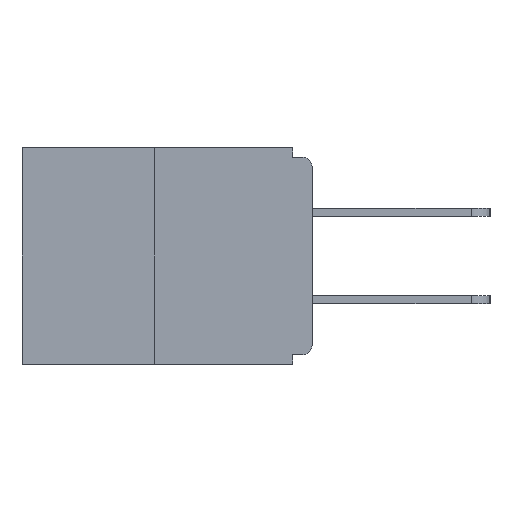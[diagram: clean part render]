
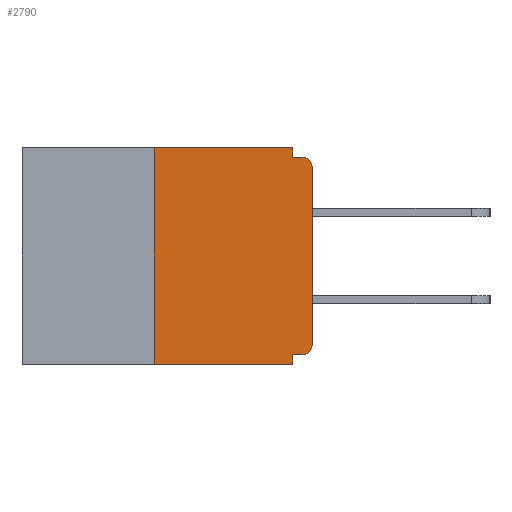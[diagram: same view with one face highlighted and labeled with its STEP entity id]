
A CAD part, left-side view. The second image highlights one B-rep face of the part: STEP entity #2790.
In plain terms, the highlighted planar face has unit normal (-1, 0, 0).
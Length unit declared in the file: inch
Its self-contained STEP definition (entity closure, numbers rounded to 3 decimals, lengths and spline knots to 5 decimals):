
#157 = CARTESIAN_POINT ( 'NONE',  ( 0., 0.25, 0. ) ) ;
#269 = EDGE_CURVE ( 'NONE', #6427, #12212, #11027, .T. ) ;
#271 = VERTEX_POINT ( 'NONE', #157 ) ;
#333 = CARTESIAN_POINT ( 'NONE',  ( 0., 0.031, -0.328 ) ) ;
#375 = DIRECTION ( 'NONE',  ( 0., 0., -1. ) ) ;
#727 = LINE ( 'NONE', #1716, #4737 ) ;
#828 = AXIS2_PLACEMENT_3D ( 'NONE', #4434, #5323, #8430 ) ;
#1005 = EDGE_CURVE ( 'NONE', #9536, #6427, #4765, .T. ) ;
#1141 = EDGE_CURVE ( 'NONE', #8520, #8448, #3304, .T. ) ;
#1332 = CARTESIAN_POINT ( 'NONE',  ( 0., 0.031, 0. ) ) ;
#1420 = DIRECTION ( 'NONE',  ( 0., -1., 0. ) ) ;
#1457 = CARTESIAN_POINT ( 'NONE',  ( 0., 0.031, 0. ) ) ;
#1528 = CARTESIAN_POINT ( 'NONE',  ( 0., 0.46, 0. ) ) ;
#1587 = DIRECTION ( 'NONE',  ( 1., 0., 0. ) ) ;
#1629 = DIRECTION ( 'NONE',  ( 0., 0., 1. ) ) ;
#1716 = CARTESIAN_POINT ( 'NONE',  ( 0., 0., 0. ) ) ;
#2136 = ORIENTED_EDGE ( 'NONE', *, *, #1141, .F. ) ;
#2219 = CARTESIAN_POINT ( 'NONE',  ( 0., 0., -0.313 ) ) ;
#2354 = DIRECTION ( 'NONE',  ( 0., 0., -1. ) ) ;
#2359 = CARTESIAN_POINT ( 'NONE',  ( 0., 0.015, -0.015 ) ) ;
#2559 = DIRECTION ( 'NONE',  ( 0., 0., -1. ) ) ;
#2600 = ORIENTED_EDGE ( 'NONE', *, *, #269, .F. ) ;
#2650 = EDGE_CURVE ( 'NONE', #9536, #10137, #5024, .T. ) ;
#2684 = VECTOR ( 'NONE', #4044, 39.37008 ) ;
#2790 = ADVANCED_FACE ( 'NONE', ( #4387 ), #12903, .F. ) ;
#3304 = LINE ( 'NONE', #1332, #8453 ) ;
#3417 = DIRECTION ( 'NONE',  ( 0., -1., 0. ) ) ;
#3632 = LINE ( 'NONE', #8275, #12004 ) ;
#3645 = CARTESIAN_POINT ( 'NONE',  ( 0., 0.031, -0.343 ) ) ;
#3971 = EDGE_CURVE ( 'NONE', #11972, #12212, #5614, .T. ) ;
#4044 = DIRECTION ( 'NONE',  ( 0., 1., 0. ) ) ;
#4387 = FACE_OUTER_BOUND ( 'NONE', #6310, .T. ) ;
#4434 = CARTESIAN_POINT ( 'NONE',  ( 0., 0.015, -0.313 ) ) ;
#4737 = VECTOR ( 'NONE', #1629, 39.37008 ) ;
#4765 = LINE ( 'NONE', #10283, #2684 ) ;
#4821 = VECTOR ( 'NONE', #3417, 39.37008 ) ;
#5024 = CIRCLE ( 'NONE', #828, 0.015 ) ;
#5153 = VECTOR ( 'NONE', #6194, 39.37008 ) ;
#5249 = VECTOR ( 'NONE', #375, 39.37008 ) ;
#5323 = DIRECTION ( 'NONE',  ( -1., 0., 0. ) ) ;
#5543 = ORIENTED_EDGE ( 'NONE', *, *, #3971, .T. ) ;
#5614 = LINE ( 'NONE', #9559, #11400 ) ;
#6194 = DIRECTION ( 'NONE',  ( 0., -1., 0. ) ) ;
#6268 = CARTESIAN_POINT ( 'NONE',  ( 0., 0., -0.03 ) ) ;
#6310 = EDGE_LOOP ( 'NONE', ( #10351, #6966, #5543, #2600, #7710, #12036, #12906, #10651, #11792, #2136 ) ) ;
#6427 = VERTEX_POINT ( 'NONE', #333 ) ;
#6457 = CARTESIAN_POINT ( 'NONE',  ( 0., 0.031, -0.015 ) ) ;
#6832 = EDGE_CURVE ( 'NONE', #11972, #271, #3632, .T. ) ;
#6966 = ORIENTED_EDGE ( 'NONE', *, *, #6832, .F. ) ;
#7224 = CARTESIAN_POINT ( 'NONE',  ( 0., 0., -0.015 ) ) ;
#7710 = ORIENTED_EDGE ( 'NONE', *, *, #1005, .F. ) ;
#7743 = CARTESIAN_POINT ( 'NONE',  ( 0., 0.25, -0.343 ) ) ;
#8275 = CARTESIAN_POINT ( 'NONE',  ( 0., 0.25, 0. ) ) ;
#8430 = DIRECTION ( 'NONE',  ( 0., 0., -1. ) ) ;
#8448 = VERTEX_POINT ( 'NONE', #6457 ) ;
#8453 = VECTOR ( 'NONE', #2354, 39.37008 ) ;
#8520 = VERTEX_POINT ( 'NONE', #1457 ) ;
#8607 = CARTESIAN_POINT ( 'NONE',  ( 0., 0.46, 0. ) ) ;
#8851 = VERTEX_POINT ( 'NONE', #2359 ) ;
#8991 = VERTEX_POINT ( 'NONE', #6268 ) ;
#9115 = EDGE_CURVE ( 'NONE', #10137, #8991, #727, .T. ) ;
#9363 = CARTESIAN_POINT ( 'NONE',  ( 0., 0.031, -0.343 ) ) ;
#9536 = VERTEX_POINT ( 'NONE', #12964 ) ;
#9559 = CARTESIAN_POINT ( 'NONE',  ( 0., 0.46, -0.343 ) ) ;
#10137 = VERTEX_POINT ( 'NONE', #2219 ) ;
#10283 = CARTESIAN_POINT ( 'NONE',  ( 0., 0., -0.328 ) ) ;
#10351 = ORIENTED_EDGE ( 'NONE', *, *, #11617, .F. ) ;
#10532 = EDGE_CURVE ( 'NONE', #8448, #8851, #11089, .T. ) ;
#10587 = DIRECTION ( 'NONE',  ( 0., 0., 1. ) ) ;
#10651 = ORIENTED_EDGE ( 'NONE', *, *, #11962, .T. ) ;
#10937 = AXIS2_PLACEMENT_3D ( 'NONE', #8607, #1587, #2559 ) ;
#11027 = LINE ( 'NONE', #9363, #5249 ) ;
#11089 = LINE ( 'NONE', #7224, #5153 ) ;
#11189 = CARTESIAN_POINT ( 'NONE',  ( 0., 0.015, -0.03 ) ) ;
#11386 = LINE ( 'NONE', #1528, #4821 ) ;
#11400 = VECTOR ( 'NONE', #1420, 39.37008 ) ;
#11617 = EDGE_CURVE ( 'NONE', #271, #8520, #11386, .T. ) ;
#11792 = ORIENTED_EDGE ( 'NONE', *, *, #10532, .F. ) ;
#11880 = CIRCLE ( 'NONE', #12660, 0.015 ) ;
#11962 = EDGE_CURVE ( 'NONE', #8991, #8851, #11880, .T. ) ;
#11972 = VERTEX_POINT ( 'NONE', #7743 ) ;
#12004 = VECTOR ( 'NONE', #10587, 39.37008 ) ;
#12036 = ORIENTED_EDGE ( 'NONE', *, *, #2650, .T. ) ;
#12205 = DIRECTION ( 'NONE',  ( 0., 0., -1. ) ) ;
#12212 = VERTEX_POINT ( 'NONE', #3645 ) ;
#12248 = DIRECTION ( 'NONE',  ( -1., 0., 0. ) ) ;
#12660 = AXIS2_PLACEMENT_3D ( 'NONE', #11189, #12248, #12205 ) ;
#12903 = PLANE ( 'NONE',  #10937 ) ;
#12906 = ORIENTED_EDGE ( 'NONE', *, *, #9115, .T. ) ;
#12964 = CARTESIAN_POINT ( 'NONE',  ( 0., 0.015, -0.328 ) ) ;
